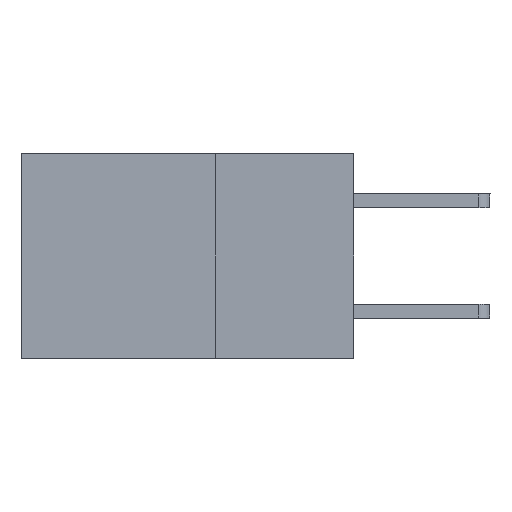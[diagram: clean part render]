
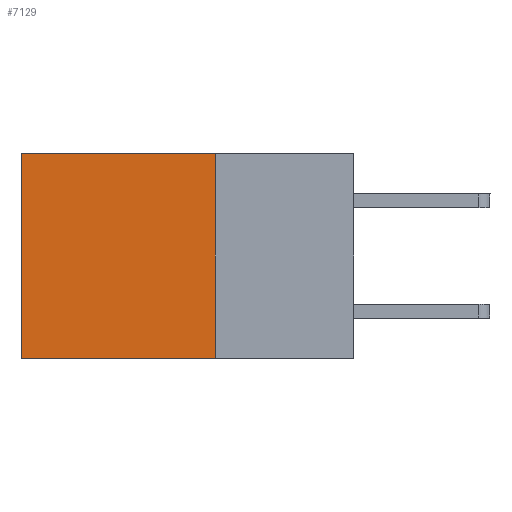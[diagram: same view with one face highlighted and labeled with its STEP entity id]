
A CAD part, left-side view. The second image highlights one B-rep face of the part: STEP entity #7129.
In plain terms, the highlighted planar face has unit normal (-1, 0, 0).
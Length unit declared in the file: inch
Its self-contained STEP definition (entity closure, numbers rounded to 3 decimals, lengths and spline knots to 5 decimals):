
#414 = PLANE ( 'NONE',  #12070 ) ;
#605 = VECTOR ( 'NONE', #9224, 39.37008 ) ;
#1471 = EDGE_CURVE ( 'NONE', #6349, #2735, #8747, .T. ) ;
#2621 = VECTOR ( 'NONE', #7963, 39.37008 ) ;
#2735 = VERTEX_POINT ( 'NONE', #11633 ) ;
#2858 = CARTESIAN_POINT ( 'NONE',  ( 0.2875, 0.25, 0. ) ) ;
#2910 = DIRECTION ( 'NONE',  ( 0., 0., -1. ) ) ;
#2912 = EDGE_LOOP ( 'NONE', ( #12160, #12388, #12430, #12446 ) ) ;
#3490 = CARTESIAN_POINT ( 'NONE',  ( 0.2875, 0.6, 0. ) ) ;
#3823 = VECTOR ( 'NONE', #7314, 39.37008 ) ;
#4005 = VERTEX_POINT ( 'NONE', #13805 ) ;
#4868 = LINE ( 'NONE', #3490, #13363 ) ;
#6135 = FACE_OUTER_BOUND ( 'NONE', #2912, .T. ) ;
#6157 = LINE ( 'NONE', #8057, #605 ) ;
#6349 = VERTEX_POINT ( 'NONE', #8914 ) ;
#6521 = EDGE_CURVE ( 'NONE', #8819, #4005, #4868, .T. ) ;
#7050 = EDGE_CURVE ( 'NONE', #2735, #4005, #12728, .T. ) ;
#7129 = ADVANCED_FACE ( 'NONE', ( #6135 ), #414, .F. ) ;
#7314 = DIRECTION ( 'NONE',  ( 0., 1., 0. ) ) ;
#7366 = CARTESIAN_POINT ( 'NONE',  ( 0.2875, 0.6, 0. ) ) ;
#7901 = CARTESIAN_POINT ( 'NONE',  ( 0.2875, 0.25, 0. ) ) ;
#7963 = DIRECTION ( 'NONE',  ( 0., 0., -1. ) ) ;
#8037 = DIRECTION ( 'NONE',  ( 0., 0., -1. ) ) ;
#8057 = CARTESIAN_POINT ( 'NONE',  ( 0.2875, 0.25, 0. ) ) ;
#8747 = LINE ( 'NONE', #7901, #2621 ) ;
#8819 = VERTEX_POINT ( 'NONE', #7366 ) ;
#8914 = CARTESIAN_POINT ( 'NONE',  ( 0.2875, 0.25, 0. ) ) ;
#9224 = DIRECTION ( 'NONE',  ( 0., 1., 0. ) ) ;
#9773 = DIRECTION ( 'NONE',  ( 1., 0., 0. ) ) ;
#11633 = CARTESIAN_POINT ( 'NONE',  ( 0.2875, 0.25, -0.37 ) ) ;
#12070 = AXIS2_PLACEMENT_3D ( 'NONE', #2858, #9773, #2910 ) ;
#12119 = EDGE_CURVE ( 'NONE', #6349, #8819, #6157, .T. ) ;
#12160 = ORIENTED_EDGE ( 'NONE', *, *, #6521, .T. ) ;
#12388 = ORIENTED_EDGE ( 'NONE', *, *, #7050, .F. ) ;
#12430 = ORIENTED_EDGE ( 'NONE', *, *, #1471, .F. ) ;
#12446 = ORIENTED_EDGE ( 'NONE', *, *, #12119, .T. ) ;
#12728 = LINE ( 'NONE', #12801, #3823 ) ;
#12801 = CARTESIAN_POINT ( 'NONE',  ( 0.2875, 0.25, -0.37 ) ) ;
#13363 = VECTOR ( 'NONE', #8037, 39.37008 ) ;
#13805 = CARTESIAN_POINT ( 'NONE',  ( 0.2875, 0.6, -0.37 ) ) ;
